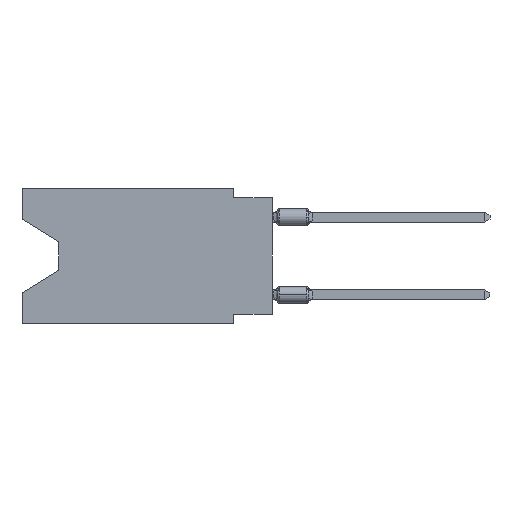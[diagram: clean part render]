
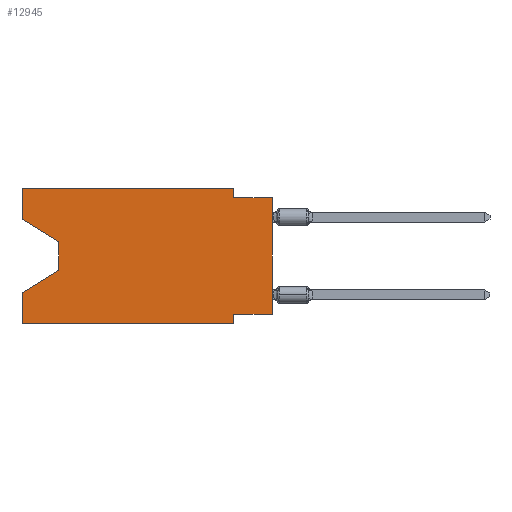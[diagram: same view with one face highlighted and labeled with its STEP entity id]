
A CAD part, left-side view. The second image highlights one B-rep face of the part: STEP entity #12945.
In plain terms, the highlighted planar face has unit normal (-1, 0, 0).
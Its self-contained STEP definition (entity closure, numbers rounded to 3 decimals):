
#341 = LINE ( 'NONE', #10904, #7782 ) ;
#509 = ORIENTED_EDGE ( 'NONE', *, *, #7011, .T. ) ;
#1179 = CARTESIAN_POINT ( 'NONE',  ( 0., 16.383, 0. ) ) ;
#1252 = CARTESIAN_POINT ( 'NONE',  ( 0., 16.383, 0. ) ) ;
#1346 = CARTESIAN_POINT ( 'NONE',  ( 0., 2.54, -8.255 ) ) ;
#1359 = EDGE_CURVE ( 'NONE', #7934, #5947, #5745, .T. ) ;
#1406 = CARTESIAN_POINT ( 'NONE',  ( 0., 0., -8.255 ) ) ;
#1581 = EDGE_CURVE ( 'NONE', #15116, #6869, #341, .T. ) ;
#1710 = VERTEX_POINT ( 'NONE', #8738 ) ;
#2026 = EDGE_CURVE ( 'NONE', #3743, #1710, #8360, .T. ) ;
#2097 = DIRECTION ( 'NONE',  ( 0., 0., 1. ) ) ;
#2491 = FACE_OUTER_BOUND ( 'NONE', #9866, .T. ) ;
#2520 = CARTESIAN_POINT ( 'NONE',  ( 0., 2.54, -8.89 ) ) ;
#2552 = VERTEX_POINT ( 'NONE', #2699 ) ;
#2630 = ORIENTED_EDGE ( 'NONE', *, *, #9761, .T. ) ;
#2699 = CARTESIAN_POINT ( 'NONE',  ( 0., 0., -8.255 ) ) ;
#2784 = ORIENTED_EDGE ( 'NONE', *, *, #6082, .T. ) ;
#3631 = VECTOR ( 'NONE', #8649, 1000. ) ;
#3743 = VERTEX_POINT ( 'NONE', #3939 ) ;
#3939 = CARTESIAN_POINT ( 'NONE',  ( 0., 16.383, -2.038 ) ) ;
#4133 = ORIENTED_EDGE ( 'NONE', *, *, #6024, .F. ) ;
#4955 = DIRECTION ( 'NONE',  ( 0., -0.855, -0.519 ) ) ;
#5110 = EDGE_CURVE ( 'NONE', #3743, #7934, #10349, .T. ) ;
#5159 = CARTESIAN_POINT ( 'NONE',  ( 0., 16.383, 0. ) ) ;
#5196 = CARTESIAN_POINT ( 'NONE',  ( 0., 0., -0.635 ) ) ;
#5660 = VECTOR ( 'NONE', #11068, 1000. ) ;
#5741 = AXIS2_PLACEMENT_3D ( 'NONE', #1179, #9585, #7344 ) ;
#5745 = LINE ( 'NONE', #9148, #10958 ) ;
#5947 = VERTEX_POINT ( 'NONE', #8386 ) ;
#6024 = EDGE_CURVE ( 'NONE', #10300, #7710, #7606, .T. ) ;
#6082 = EDGE_CURVE ( 'NONE', #12155, #6456, #8603, .T. ) ;
#6387 = VECTOR ( 'NONE', #14138, 1000. ) ;
#6456 = VERTEX_POINT ( 'NONE', #12049 ) ;
#6748 = ORIENTED_EDGE ( 'NONE', *, *, #7114, .F. ) ;
#6761 = CARTESIAN_POINT ( 'NONE',  ( 0., 2.54, 0. ) ) ;
#6869 = VERTEX_POINT ( 'NONE', #13616 ) ;
#6886 = VECTOR ( 'NONE', #11173, 1000. ) ;
#6898 = CARTESIAN_POINT ( 'NONE',  ( 0., 16.383, -8.89 ) ) ;
#6923 = LINE ( 'NONE', #2520, #6387 ) ;
#7011 = EDGE_CURVE ( 'NONE', #2552, #7710, #7930, .T. ) ;
#7090 = VECTOR ( 'NONE', #14333, 1000. ) ;
#7114 = EDGE_CURVE ( 'NONE', #9418, #6456, #6923, .T. ) ;
#7345 = CARTESIAN_POINT ( 'NONE',  ( 0., 13.97, -3.505 ) ) ;
#7344 = DIRECTION ( 'NONE',  ( 0., 0., -1. ) ) ;
#7606 = LINE ( 'NONE', #10985, #5660 ) ;
#7710 = VERTEX_POINT ( 'NONE', #5196 ) ;
#7782 = VECTOR ( 'NONE', #11978, 1000. ) ;
#7930 = LINE ( 'NONE', #15070, #8879 ) ;
#7934 = VERTEX_POINT ( 'NONE', #1252 ) ;
#7960 = CARTESIAN_POINT ( 'NONE',  ( 0., 16.383, 0. ) ) ;
#8004 = DIRECTION ( 'NONE',  ( 0., 0., 1. ) ) ;
#8360 = LINE ( 'NONE', #13118, #12694 ) ;
#8386 = CARTESIAN_POINT ( 'NONE',  ( 0., 2.54, 0. ) ) ;
#8603 = LINE ( 'NONE', #13290, #12294 ) ;
#8649 = DIRECTION ( 'NONE',  ( 0., 1., 0. ) ) ;
#8738 = CARTESIAN_POINT ( 'NONE',  ( 0., 13.97, -3.505 ) ) ;
#8879 = VECTOR ( 'NONE', #8004, 1000. ) ;
#9148 = CARTESIAN_POINT ( 'NONE',  ( 0., 16.383, 0. ) ) ;
#9214 = DIRECTION ( 'NONE',  ( 0., -1., 0. ) ) ;
#9395 = ORIENTED_EDGE ( 'NONE', *, *, #5110, .F. ) ;
#9418 = VERTEX_POINT ( 'NONE', #1346 ) ;
#9585 = DIRECTION ( 'NONE',  ( 1., 0., 0. ) ) ;
#9659 = LINE ( 'NONE', #1406, #3631 ) ;
#9669 = VECTOR ( 'NONE', #14995, 1000. ) ;
#9761 = EDGE_CURVE ( 'NONE', #1710, #15116, #10886, .T. ) ;
#9779 = EDGE_CURVE ( 'NONE', #2552, #9418, #9659, .T. ) ;
#9783 = LINE ( 'NONE', #5159, #6886 ) ;
#9866 = EDGE_LOOP ( 'NONE', ( #12602, #2630, #13399, #13036, #2784, #6748, #13855, #509, #4133, #10076, #10608, #9395 ) ) ;
#10076 = ORIENTED_EDGE ( 'NONE', *, *, #14044, .F. ) ;
#10300 = VERTEX_POINT ( 'NONE', #15062 ) ;
#10349 = LINE ( 'NONE', #7960, #11296 ) ;
#10608 = ORIENTED_EDGE ( 'NONE', *, *, #1359, .F. ) ;
#10886 = LINE ( 'NONE', #7345, #7090 ) ;
#10885 = PLANE ( 'NONE',  #5741 ) ;
#10904 = CARTESIAN_POINT ( 'NONE',  ( 0., 13.97, -5.385 ) ) ;
#10958 = VECTOR ( 'NONE', #12833, 1000. ) ;
#10985 = CARTESIAN_POINT ( 'NONE',  ( 0., 0., -0.635 ) ) ;
#11068 = DIRECTION ( 'NONE',  ( 0., -1., 0. ) ) ;
#11173 = DIRECTION ( 'NONE',  ( 0., 0., 1. ) ) ;
#11296 = VECTOR ( 'NONE', #2097, 1000. ) ;
#11978 = DIRECTION ( 'NONE',  ( 0., 0.855, -0.519 ) ) ;
#12049 = CARTESIAN_POINT ( 'NONE',  ( 0., 2.54, -8.89 ) ) ;
#12155 = VERTEX_POINT ( 'NONE', #6898 ) ;
#12235 = CARTESIAN_POINT ( 'NONE',  ( 0., 13.97, -5.385 ) ) ;
#12294 = VECTOR ( 'NONE', #9214, 1000. ) ;
#12561 = EDGE_CURVE ( 'NONE', #12155, #6869, #9783, .T. ) ;
#12602 = ORIENTED_EDGE ( 'NONE', *, *, #2026, .T. ) ;
#12694 = VECTOR ( 'NONE', #4955, 1000. ) ;
#12833 = DIRECTION ( 'NONE',  ( 0., -1., 0. ) ) ;
#12945 = ADVANCED_FACE ( 'NONE', ( #2491 ), #10885, .F. ) ;
#13036 = ORIENTED_EDGE ( 'NONE', *, *, #12561, .F. ) ;
#13118 = CARTESIAN_POINT ( 'NONE',  ( 0., 16.383, -2.038 ) ) ;
#13290 = CARTESIAN_POINT ( 'NONE',  ( 0., 16.383, -8.89 ) ) ;
#13399 = ORIENTED_EDGE ( 'NONE', *, *, #1581, .T. ) ;
#13616 = CARTESIAN_POINT ( 'NONE',  ( 0., 16.383, -6.852 ) ) ;
#13833 = LINE ( 'NONE', #6761, #9669 ) ;
#13855 = ORIENTED_EDGE ( 'NONE', *, *, #9779, .F. ) ;
#14044 = EDGE_CURVE ( 'NONE', #5947, #10300, #13833, .T. ) ;
#14138 = DIRECTION ( 'NONE',  ( 0., 0., -1. ) ) ;
#14333 = DIRECTION ( 'NONE',  ( 0., 0., -1. ) ) ;
#14995 = DIRECTION ( 'NONE',  ( 0., 0., -1. ) ) ;
#15062 = CARTESIAN_POINT ( 'NONE',  ( 0., 2.54, -0.635 ) ) ;
#15070 = CARTESIAN_POINT ( 'NONE',  ( 0., 0., 0. ) ) ;
#15116 = VERTEX_POINT ( 'NONE', #12235 ) ;
